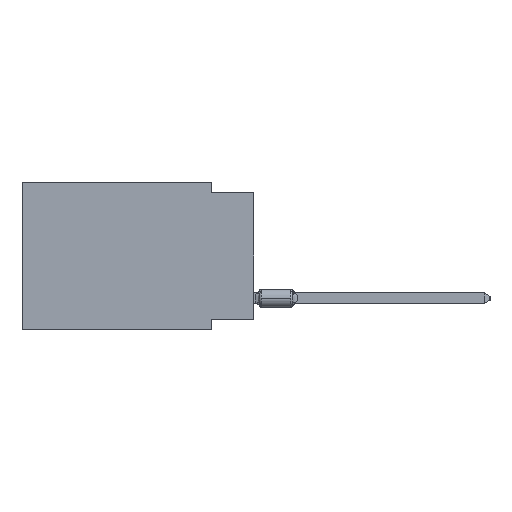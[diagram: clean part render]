
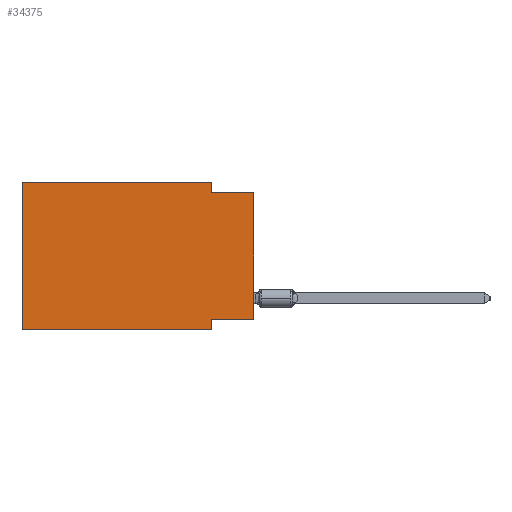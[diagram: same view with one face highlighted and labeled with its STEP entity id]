
A CAD part, left-side view. The second image highlights one B-rep face of the part: STEP entity #34375.
In plain terms, the highlighted planar face has unit normal (-1, 0, 0).
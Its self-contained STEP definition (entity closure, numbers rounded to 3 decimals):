
#928 = VERTEX_POINT ( 'NONE', #28754 ) ;
#2458 = EDGE_CURVE ( 'NONE', #10973, #8052, #34958, .T. ) ;
#2804 = EDGE_CURVE ( 'NONE', #10973, #15895, #28280, .T. ) ;
#3580 = VECTOR ( 'NONE', #34789, 1000. ) ;
#3718 = EDGE_CURVE ( 'NONE', #13197, #10821, #4038, .T. ) ;
#4038 = LINE ( 'NONE', #20578, #26149 ) ;
#4311 = EDGE_CURVE ( 'NONE', #15895, #23115, #13259, .T. ) ;
#4553 = VECTOR ( 'NONE', #8210, 1000. ) ;
#4917 = CARTESIAN_POINT ( 'NONE',  ( 0., 2.54, 0. ) ) ;
#7049 = CARTESIAN_POINT ( 'NONE',  ( 0., 0., -8.255 ) ) ;
#7349 = ORIENTED_EDGE ( 'NONE', *, *, #24223, .F. ) ;
#7504 = CARTESIAN_POINT ( 'NONE',  ( 0., 13.97, -8.89 ) ) ;
#8052 = VERTEX_POINT ( 'NONE', #32942 ) ;
#8210 = DIRECTION ( 'NONE',  ( 0., -1., 0. ) ) ;
#9427 = VECTOR ( 'NONE', #24667, 1000. ) ;
#10408 = ORIENTED_EDGE ( 'NONE', *, *, #28212, .T. ) ;
#10416 = DIRECTION ( 'NONE',  ( 0., -1., 0. ) ) ;
#10821 = VERTEX_POINT ( 'NONE', #17063 ) ;
#10973 = VERTEX_POINT ( 'NONE', #7504 ) ;
#12316 = DIRECTION ( 'NONE',  ( 0., 0., -1. ) ) ;
#13093 = LINE ( 'NONE', #4917, #9427 ) ;
#13197 = VERTEX_POINT ( 'NONE', #29830 ) ;
#13259 = LINE ( 'NONE', #36417, #34804 ) ;
#13881 = VECTOR ( 'NONE', #20900, 1000. ) ;
#15895 = VERTEX_POINT ( 'NONE', #16755 ) ;
#16214 = EDGE_LOOP ( 'NONE', ( #10408, #37228, #28963, #36602, #29824, #17045, #7349, #29614 ) ) ;
#16755 = CARTESIAN_POINT ( 'NONE',  ( 0., 13.97, 0. ) ) ;
#16946 = LINE ( 'NONE', #25865, #3580 ) ;
#17045 = ORIENTED_EDGE ( 'NONE', *, *, #2458, .T. ) ;
#17063 = CARTESIAN_POINT ( 'NONE',  ( 0., 0., -0.635 ) ) ;
#17100 = DIRECTION ( 'NONE',  ( 0., 0., 1. ) ) ;
#18293 = AXIS2_PLACEMENT_3D ( 'NONE', #18749, #32427, #12316 ) ;
#18390 = FACE_OUTER_BOUND ( 'NONE', #16214, .T. ) ;
#18749 = CARTESIAN_POINT ( 'NONE',  ( 0., 13.97, 0. ) ) ;
#20132 = CARTESIAN_POINT ( 'NONE',  ( 0., 0., 0. ) ) ;
#20578 = CARTESIAN_POINT ( 'NONE',  ( 0., 0., -0.635 ) ) ;
#20900 = DIRECTION ( 'NONE',  ( 0., 1., 0. ) ) ;
#21578 = VERTEX_POINT ( 'NONE', #33654 ) ;
#23115 = VERTEX_POINT ( 'NONE', #26812 ) ;
#24223 = EDGE_CURVE ( 'NONE', #928, #8052, #16946, .T. ) ;
#24667 = DIRECTION ( 'NONE',  ( 0., 0., -1. ) ) ;
#25433 = DIRECTION ( 'NONE',  ( 0., 0., 1. ) ) ;
#25865 = CARTESIAN_POINT ( 'NONE',  ( 0., 2.54, -8.89 ) ) ;
#26149 = VECTOR ( 'NONE', #35927, 1000. ) ;
#26430 = VECTOR ( 'NONE', #17100, 1000. ) ;
#26812 = CARTESIAN_POINT ( 'NONE',  ( 0., 2.54, 0. ) ) ;
#26850 = EDGE_CURVE ( 'NONE', #23115, #13197, #13093, .T. ) ;
#27290 = PLANE ( 'NONE',  #18293 ) ;
#28212 = EDGE_CURVE ( 'NONE', #21578, #10821, #28481, .T. ) ;
#28280 = LINE ( 'NONE', #37213, #35466 ) ;
#28481 = LINE ( 'NONE', #20132, #26430 ) ;
#28754 = CARTESIAN_POINT ( 'NONE',  ( 0., 2.54, -8.255 ) ) ;
#28963 = ORIENTED_EDGE ( 'NONE', *, *, #26850, .F. ) ;
#29614 = ORIENTED_EDGE ( 'NONE', *, *, #31577, .F. ) ;
#29824 = ORIENTED_EDGE ( 'NONE', *, *, #2804, .F. ) ;
#29830 = CARTESIAN_POINT ( 'NONE',  ( 0., 2.54, -0.635 ) ) ;
#30021 = LINE ( 'NONE', #7049, #13881 ) ;
#31366 = CARTESIAN_POINT ( 'NONE',  ( 0., 13.97, -8.89 ) ) ;
#31577 = EDGE_CURVE ( 'NONE', #21578, #928, #30021, .T. ) ;
#32427 = DIRECTION ( 'NONE',  ( 1., 0., 0. ) ) ;
#32942 = CARTESIAN_POINT ( 'NONE',  ( 0., 2.54, -8.89 ) ) ;
#33654 = CARTESIAN_POINT ( 'NONE',  ( 0., 0., -8.255 ) ) ;
#34375 = ADVANCED_FACE ( 'NONE', ( #18390 ), #27290, .F. ) ;
#34789 = DIRECTION ( 'NONE',  ( 0., 0., -1. ) ) ;
#34804 = VECTOR ( 'NONE', #10416, 1000. ) ;
#34958 = LINE ( 'NONE', #31366, #4553 ) ;
#35466 = VECTOR ( 'NONE', #25433, 1000. ) ;
#35927 = DIRECTION ( 'NONE',  ( 0., -1., 0. ) ) ;
#36417 = CARTESIAN_POINT ( 'NONE',  ( 0., 13.97, 0. ) ) ;
#36602 = ORIENTED_EDGE ( 'NONE', *, *, #4311, .F. ) ;
#37213 = CARTESIAN_POINT ( 'NONE',  ( 0., 13.97, 0. ) ) ;
#37228 = ORIENTED_EDGE ( 'NONE', *, *, #3718, .F. ) ;
